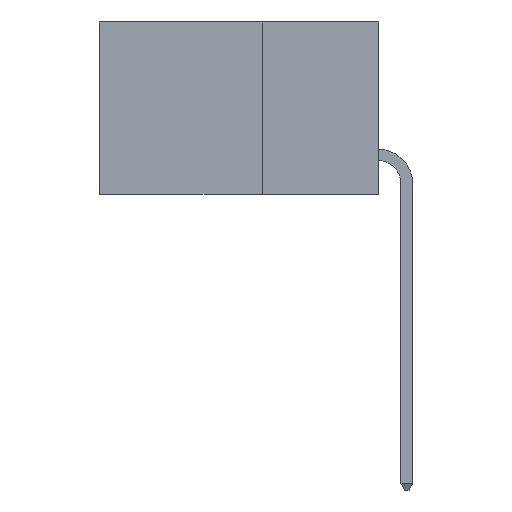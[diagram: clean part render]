
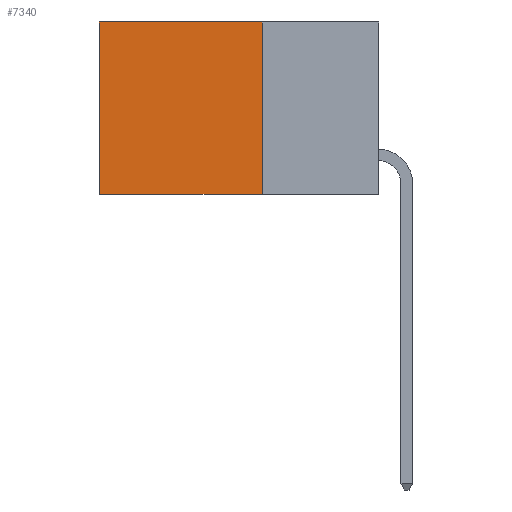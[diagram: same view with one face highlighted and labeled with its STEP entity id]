
A CAD part, left-side view. The second image highlights one B-rep face of the part: STEP entity #7340.
In plain terms, the highlighted planar face has unit normal (-1, 0, 0).
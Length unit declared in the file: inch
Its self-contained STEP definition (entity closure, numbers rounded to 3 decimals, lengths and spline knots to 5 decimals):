
#231 = DIRECTION ( 'NONE',  ( 0., 1., 0. ) ) ;
#267 = VECTOR ( 'NONE', #231, 39.37008 ) ;
#678 = EDGE_CURVE ( 'NONE', #901, #7887, #5968, .T. ) ;
#901 = VERTEX_POINT ( 'NONE', #9880 ) ;
#1511 = VERTEX_POINT ( 'NONE', #9160 ) ;
#1696 = DIRECTION ( 'NONE',  ( 0., 1., 0. ) ) ;
#1727 = CARTESIAN_POINT ( 'NONE',  ( 0.2615, 0.25, -0.37 ) ) ;
#2320 = ORIENTED_EDGE ( 'NONE', *, *, #678, .T. ) ;
#2331 = ORIENTED_EDGE ( 'NONE', *, *, #8991, .F. ) ;
#2352 = ORIENTED_EDGE ( 'NONE', *, *, #7664, .F. ) ;
#2355 = ORIENTED_EDGE ( 'NONE', *, *, #6768, .T. ) ;
#3059 = LINE ( 'NONE', #4368, #267 ) ;
#3320 = DIRECTION ( 'NONE',  ( 0., 0., -1. ) ) ;
#3439 = VECTOR ( 'NONE', #10882, 39.37008 ) ;
#3667 = CARTESIAN_POINT ( 'NONE',  ( 0.2615, 0.6, -0.37 ) ) ;
#4368 = CARTESIAN_POINT ( 'NONE',  ( 0.2615, 0.25, -0.37 ) ) ;
#4678 = VERTEX_POINT ( 'NONE', #8162 ) ;
#4684 = AXIS2_PLACEMENT_3D ( 'NONE', #1727, #5723, #11788 ) ;
#5092 = LINE ( 'NONE', #6566, #7163 ) ;
#5723 = DIRECTION ( 'NONE',  ( 1., 0., 0. ) ) ;
#5787 = VECTOR ( 'NONE', #3320, 39.37008 ) ;
#5968 = LINE ( 'NONE', #11938, #3439 ) ;
#6566 = CARTESIAN_POINT ( 'NONE',  ( 0.2615, 0.25, 0. ) ) ;
#6768 = EDGE_CURVE ( 'NONE', #4678, #901, #5092, .T. ) ;
#7023 = FACE_OUTER_BOUND ( 'NONE', #9113, .T. ) ;
#7163 = VECTOR ( 'NONE', #1696, 39.37008 ) ;
#7340 = ADVANCED_FACE ( 'NONE', ( #7023 ), #8326, .F. ) ;
#7664 = EDGE_CURVE ( 'NONE', #4678, #1511, #8379, .T. ) ;
#7881 = CARTESIAN_POINT ( 'NONE',  ( 0.2615, 0.25, -0.37 ) ) ;
#7887 = VERTEX_POINT ( 'NONE', #3667 ) ;
#8162 = CARTESIAN_POINT ( 'NONE',  ( 0.2615, 0.25, 0. ) ) ;
#8326 = PLANE ( 'NONE',  #4684 ) ;
#8379 = LINE ( 'NONE', #7881, #5787 ) ;
#8991 = EDGE_CURVE ( 'NONE', #1511, #7887, #3059, .T. ) ;
#9113 = EDGE_LOOP ( 'NONE', ( #2320, #2331, #2352, #2355 ) ) ;
#9160 = CARTESIAN_POINT ( 'NONE',  ( 0.2615, 0.25, -0.37 ) ) ;
#9880 = CARTESIAN_POINT ( 'NONE',  ( 0.2615, 0.6, 0. ) ) ;
#10882 = DIRECTION ( 'NONE',  ( 0., 0., -1. ) ) ;
#11788 = DIRECTION ( 'NONE',  ( 0., 0., -1. ) ) ;
#11938 = CARTESIAN_POINT ( 'NONE',  ( 0.2615, 0.6, -0.37 ) ) ;
